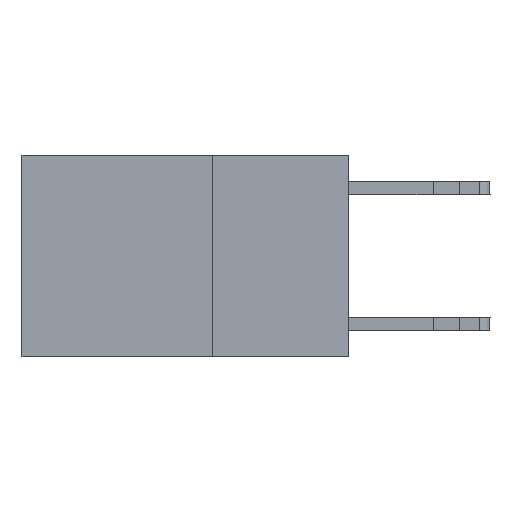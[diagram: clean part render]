
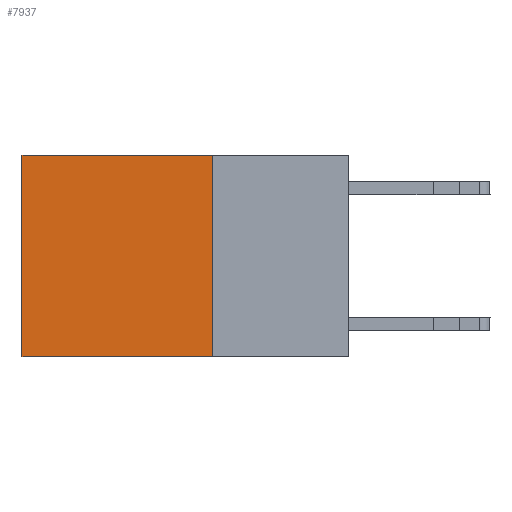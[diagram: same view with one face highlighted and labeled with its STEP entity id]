
A CAD part, left-side view. The second image highlights one B-rep face of the part: STEP entity #7937.
In plain terms, the highlighted planar face has unit normal (-1, 0, 0).
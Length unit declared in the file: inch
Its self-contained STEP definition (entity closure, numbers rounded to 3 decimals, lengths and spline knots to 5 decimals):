
#238 = VERTEX_POINT ( 'NONE', #410 ) ;
#410 = CARTESIAN_POINT ( 'NONE',  ( 0.2625, 0.6, -0.37 ) ) ;
#867 = DIRECTION ( 'NONE',  ( 1., 0., 0. ) ) ;
#1447 = VERTEX_POINT ( 'NONE', #13020 ) ;
#2891 = LINE ( 'NONE', #21033, #14292 ) ;
#3191 = VERTEX_POINT ( 'NONE', #6783 ) ;
#4135 = LINE ( 'NONE', #7451, #16345 ) ;
#4724 = CARTESIAN_POINT ( 'NONE',  ( 0.2625, 0.25, -0.37 ) ) ;
#4753 = ORIENTED_EDGE ( 'NONE', *, *, #6302, .F. ) ;
#5647 = PLANE ( 'NONE',  #16464 ) ;
#6302 = EDGE_CURVE ( 'NONE', #16579, #238, #2891, .T. ) ;
#6589 = DIRECTION ( 'NONE',  ( 0., 1., 0. ) ) ;
#6603 = EDGE_CURVE ( 'NONE', #3191, #238, #4135, .T. ) ;
#6756 = CARTESIAN_POINT ( 'NONE',  ( 0.2625, 0.25, 0. ) ) ;
#6783 = CARTESIAN_POINT ( 'NONE',  ( 0.2625, 0.6, 0. ) ) ;
#7451 = CARTESIAN_POINT ( 'NONE',  ( 0.2625, 0.6, 0. ) ) ;
#7554 = ORIENTED_EDGE ( 'NONE', *, *, #8153, .T. ) ;
#7937 = ADVANCED_FACE ( 'NONE', ( #14072 ), #5647, .F. ) ;
#8153 = EDGE_CURVE ( 'NONE', #1447, #3191, #12913, .T. ) ;
#8214 = DIRECTION ( 'NONE',  ( 0., 1., 0. ) ) ;
#8241 = EDGE_LOOP ( 'NONE', ( #20171, #4753, #12965, #7554 ) ) ;
#10397 = VECTOR ( 'NONE', #6589, 39.37008 ) ;
#12913 = LINE ( 'NONE', #19291, #10397 ) ;
#12965 = ORIENTED_EDGE ( 'NONE', *, *, #19298, .F. ) ;
#13020 = CARTESIAN_POINT ( 'NONE',  ( 0.2625, 0.25, 0. ) ) ;
#13868 = DIRECTION ( 'NONE',  ( 0., 0., -1. ) ) ;
#14072 = FACE_OUTER_BOUND ( 'NONE', #8241, .T. ) ;
#14292 = VECTOR ( 'NONE', #8214, 39.37008 ) ;
#16345 = VECTOR ( 'NONE', #20497, 39.37008 ) ;
#16464 = AXIS2_PLACEMENT_3D ( 'NONE', #17260, #867, #13868 ) ;
#16579 = VERTEX_POINT ( 'NONE', #4724 ) ;
#17260 = CARTESIAN_POINT ( 'NONE',  ( 0.2625, 0.25, 0. ) ) ;
#17953 = DIRECTION ( 'NONE',  ( 0., 0., -1. ) ) ;
#18158 = VECTOR ( 'NONE', #17953, 39.37008 ) ;
#19291 = CARTESIAN_POINT ( 'NONE',  ( 0.2625, 0.25, 0. ) ) ;
#19298 = EDGE_CURVE ( 'NONE', #1447, #16579, #19677, .T. ) ;
#19677 = LINE ( 'NONE', #6756, #18158 ) ;
#20171 = ORIENTED_EDGE ( 'NONE', *, *, #6603, .T. ) ;
#20497 = DIRECTION ( 'NONE',  ( 0., 0., -1. ) ) ;
#21033 = CARTESIAN_POINT ( 'NONE',  ( 0.2625, 0.25, -0.37 ) ) ;
